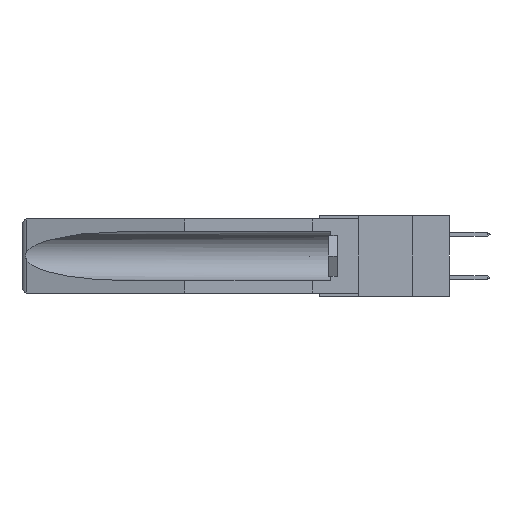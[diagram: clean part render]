
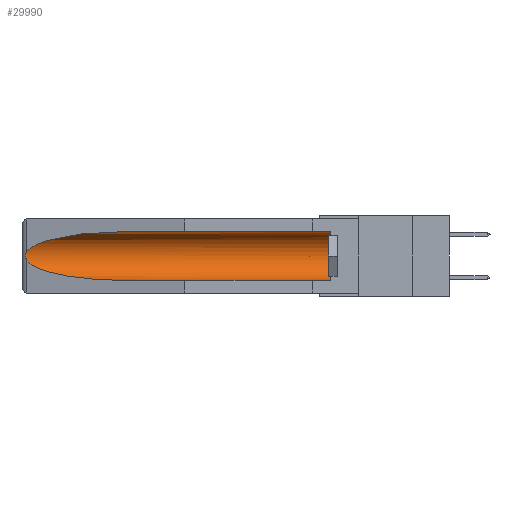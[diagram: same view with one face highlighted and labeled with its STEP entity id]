
A CAD part, left-side view. The second image highlights one B-rep face of the part: STEP entity #29990.
In plain terms, the highlighted cylindrical face has radius 2.857 mm (diameter 5.715 mm), a partial arc.
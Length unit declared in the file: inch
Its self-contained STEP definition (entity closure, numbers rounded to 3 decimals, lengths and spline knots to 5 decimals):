
#1625 = CARTESIAN_POINT ( 'NONE',  ( 0.2673, 1.5327, -0.16383 ) ) ;
#1720 = AXIS2_PLACEMENT_3D ( 'NONE', #27183, #19014, #21785 ) ;
#1976 = CARTESIAN_POINT ( 'NONE',  ( 0.155, -0.30754, -0.284 ) ) ;
#3676 = CARTESIAN_POINT ( 'NONE',  ( 0.25451, 1.48313, -0.09465 ) ) ;
#4502 = CARTESIAN_POINT ( 'NONE',  ( 0.155, 1.07973, -0.059 ) ) ;
#5667 = EDGE_CURVE ( 'NONE', #14268, #12431, #34342, .T. ) ;
#6176 = EDGE_CURVE ( 'NONE', #29542, #14840, #6906, .T. ) ;
#6619 = ORIENTED_EDGE ( 'NONE', *, *, #6176, .T. ) ;
#6639 = CARTESIAN_POINT ( 'NONE',  ( 0.26537, 1.52718, -0.19328 ) ) ;
#6906 = CIRCLE ( 'NONE', #1720, 0.1125 ) ;
#6987 = CARTESIAN_POINT ( 'NONE',  ( 0.26537, 1.52718, -0.14972 ) ) ;
#9015 = CARTESIAN_POINT ( 'NONE',  ( 0.25451, 1.48313, -0.24835 ) ) ;
#9778 = CARTESIAN_POINT ( 'NONE',  ( 0.155, -0.30754, -0.1715 ) ) ;
#10069 = CARTESIAN_POINT ( 'NONE',  ( 0.26654, 1.53092, -0.15636 ) ) ;
#10675 = ORIENTED_EDGE ( 'NONE', *, *, #11172, .T. ) ;
#11160 = DIRECTION ( 'NONE',  ( 0., 1., 0. ) ) ;
#11169 = VECTOR ( 'NONE', #26527, 39.37008 ) ;
#11172 = EDGE_CURVE ( 'NONE', #24918, #13162, #20072, .T. ) ;
#11252 = ORIENTED_EDGE ( 'NONE', *, *, #18116, .F. ) ;
#12431 = VERTEX_POINT ( 'NONE', #25946 ) ;
#12545 = CARTESIAN_POINT ( 'NONE',  ( 0.26537, 1.52718, -0.19328 ) ) ;
#12733 = DIRECTION ( 'NONE',  ( 0., 1., 0. ) ) ;
#13162 = VERTEX_POINT ( 'NONE', #14443 ) ;
#14268 = VERTEX_POINT ( 'NONE', #6639 ) ;
#14443 = CARTESIAN_POINT ( 'NONE',  ( 0.26537, 1.52718, -0.14972 ) ) ;
#14573 = CARTESIAN_POINT ( 'NONE',  ( 0.26537, 1.52718, -0.14972 ) ) ;
#14840 = VERTEX_POINT ( 'NONE', #35271 ) ;
#15036 = CARTESIAN_POINT ( 'NONE',  ( 0.26597, 1.52961, -0.15275 ) ) ;
#15518 = CARTESIAN_POINT ( 'NONE',  ( 0.2673, 1.53269, -0.17917 ) ) ;
#16879 = CARTESIAN_POINT ( 'NONE',  ( 0.26537, 1.52718, -0.19328 ) ) ;
#17568 = CARTESIAN_POINT ( 'NONE',  ( 0.155, 1.07973, -0.059 ) ) ;
#17793 = CARTESIAN_POINT ( 'NONE',  ( 0.2675, 1.53308, -0.17534 ) ) ;
#18116 = EDGE_CURVE ( 'NONE', #29542, #12431, #28688, .T. ) ;
#18298 = LINE ( 'NONE', #27534, #33701 ) ;
#19014 = DIRECTION ( 'NONE',  ( 0., -1., 0. ) ) ;
#19825 = FACE_OUTER_BOUND ( 'NONE', #26188, .T. ) ;
#20072 =( BOUNDED_CURVE ( )  B_SPLINE_CURVE ( 3, ( #17568, #23070, #3676, #14573 ),
 .UNSPECIFIED., .F., .F. ) 
 B_SPLINE_CURVE_WITH_KNOTS ( ( 4, 4 ),
 ( 4.71239, 6.08839 ),
 .UNSPECIFIED. ) 
 CURVE ( )  GEOMETRIC_REPRESENTATION_ITEM ( )  RATIONAL_B_SPLINE_CURVE ( ( 1., 0.848, 0.848, 1. ) ) 
 REPRESENTATION_ITEM ( '' )  );
#21785 = DIRECTION ( 'NONE',  ( 0., 0., 1. ) ) ;
#22386 = CARTESIAN_POINT ( 'NONE',  ( 0.155, 1.07973, -0.284 ) ) ;
#22923 = ORIENTED_EDGE ( 'NONE', *, *, #5667, .T. ) ;
#23070 = CARTESIAN_POINT ( 'NONE',  ( 0.21114, 1.30732, -0.059 ) ) ;
#23608 = DIRECTION ( 'NONE',  ( 0., 0., 1. ) ) ;
#24648 = ORIENTED_EDGE ( 'NONE', *, *, #33164, .T. ) ;
#24918 = VERTEX_POINT ( 'NONE', #4502 ) ;
#25946 = CARTESIAN_POINT ( 'NONE',  ( 0.155, 1.07973, -0.284 ) ) ;
#26188 = EDGE_LOOP ( 'NONE', ( #10675, #24648, #22923, #11252, #6619, #31557 ) ) ;
#26466 = AXIS2_PLACEMENT_3D ( 'NONE', #9778, #12733, #23608 ) ;
#26527 = DIRECTION ( 'NONE',  ( 0., 1., 0. ) ) ;
#27183 = CARTESIAN_POINT ( 'NONE',  ( 0.155, 0.126, -0.1715 ) ) ;
#27534 = CARTESIAN_POINT ( 'NONE',  ( 0.155, -0.30754, -0.059 ) ) ;
#28098 = EDGE_CURVE ( 'NONE', #14840, #24918, #18298, .T. ) ;
#28688 = LINE ( 'NONE', #1976, #11169 ) ;
#28926 = CARTESIAN_POINT ( 'NONE',  ( 0.26655, 1.53094, -0.18657 ) ) ;
#29542 = VERTEX_POINT ( 'NONE', #33687 ) ;
#29990 = ADVANCED_FACE ( 'NONE', ( #19825 ), #30564, .F. ) ;
#30564 = CYLINDRICAL_SURFACE ( 'NONE', #26466, 0.1125 ) ;
#31557 = ORIENTED_EDGE ( 'NONE', *, *, #28098, .T. ) ;
#31916 = CARTESIAN_POINT ( 'NONE',  ( 0.2675, 1.53308, -0.16763 ) ) ;
#33164 = EDGE_CURVE ( 'NONE', #13162, #14268, #33275, .T. ) ;
#33275 = B_SPLINE_CURVE_WITH_KNOTS ( 'NONE', 3,
 ( #6987, #15036, #10069, #1625, #31916, #17793, #15518, #28926, #34532, #12545 ),
 .UNSPECIFIED., .F., .F.,
 ( 4, 2, 2, 2, 4 ),
 ( 0., 0.00029, 0.00058, 0.00087, 0.00117 ),
 .UNSPECIFIED. ) ;
#33610 = CARTESIAN_POINT ( 'NONE',  ( 0.21114, 1.30732, -0.284 ) ) ;
#33687 = CARTESIAN_POINT ( 'NONE',  ( 0.155, 0.126, -0.284 ) ) ;
#33701 = VECTOR ( 'NONE', #11160, 39.37008 ) ;
#34342 =( BOUNDED_CURVE ( )  B_SPLINE_CURVE ( 3, ( #16879, #9015, #33610, #22386 ),
 .UNSPECIFIED., .F., .F. ) 
 B_SPLINE_CURVE_WITH_KNOTS ( ( 4, 4 ),
 ( 0.1948, 1.5708 ),
 .UNSPECIFIED. ) 
 CURVE ( )  GEOMETRIC_REPRESENTATION_ITEM ( )  RATIONAL_B_SPLINE_CURVE ( ( 1., 0.848, 0.848, 1. ) ) 
 REPRESENTATION_ITEM ( '' )  );
#34532 = CARTESIAN_POINT ( 'NONE',  ( 0.26597, 1.5296, -0.19026 ) ) ;
#35271 = CARTESIAN_POINT ( 'NONE',  ( 0.155, 0.126, -0.059 ) ) ;
